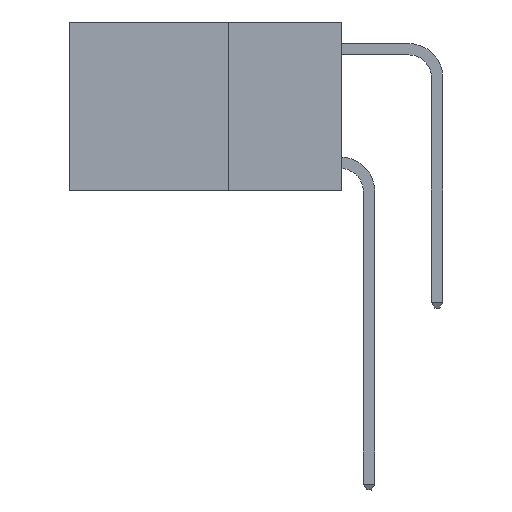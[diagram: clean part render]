
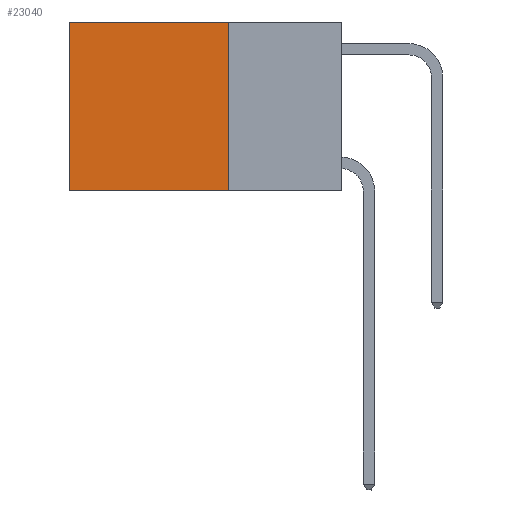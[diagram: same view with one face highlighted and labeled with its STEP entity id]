
A CAD part, left-side view. The second image highlights one B-rep face of the part: STEP entity #23040.
In plain terms, the highlighted planar face has unit normal (-1, 0, 0).
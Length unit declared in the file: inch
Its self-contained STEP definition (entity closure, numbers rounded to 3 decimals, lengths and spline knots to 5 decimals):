
#12 = VECTOR ( 'NONE', #2665, 39.37008 ) ;
#282 = ORIENTED_EDGE ( 'NONE', *, *, #5734, .F. ) ;
#461 = CARTESIAN_POINT ( 'NONE',  ( 0.2625, 0.25, 0. ) ) ;
#656 = CARTESIAN_POINT ( 'NONE',  ( 0.2625, 0.6, 0. ) ) ;
#1303 = LINE ( 'NONE', #15928, #11339 ) ;
#1490 = PLANE ( 'NONE',  #4434 ) ;
#1645 = DIRECTION ( 'NONE',  ( 0., 1., 0. ) ) ;
#2469 = DIRECTION ( 'NONE',  ( 0., 0., -1. ) ) ;
#2665 = DIRECTION ( 'NONE',  ( 0., 0., -1. ) ) ;
#3499 = DIRECTION ( 'NONE',  ( 1., 0., 0. ) ) ;
#4025 = LINE ( 'NONE', #25321, #8783 ) ;
#4434 = AXIS2_PLACEMENT_3D ( 'NONE', #15422, #3499, #17405 ) ;
#4719 = EDGE_CURVE ( 'NONE', #8634, #23724, #15917, .T. ) ;
#5163 = VECTOR ( 'NONE', #2469, 39.37008 ) ;
#5345 = CARTESIAN_POINT ( 'NONE',  ( 0.2625, 0.6, -0.37 ) ) ;
#5734 = EDGE_CURVE ( 'NONE', #16293, #23724, #4025, .T. ) ;
#6446 = LINE ( 'NONE', #461, #5163 ) ;
#8358 = EDGE_LOOP ( 'NONE', ( #12036, #282, #9505, #20150 ) ) ;
#8634 = VERTEX_POINT ( 'NONE', #14025 ) ;
#8783 = VECTOR ( 'NONE', #1645, 39.37008 ) ;
#9505 = ORIENTED_EDGE ( 'NONE', *, *, #22695, .F. ) ;
#11339 = VECTOR ( 'NONE', #13862, 39.37008 ) ;
#12036 = ORIENTED_EDGE ( 'NONE', *, *, #4719, .T. ) ;
#13862 = DIRECTION ( 'NONE',  ( 0., 1., 0. ) ) ;
#14025 = CARTESIAN_POINT ( 'NONE',  ( 0.2625, 0.6, 0. ) ) ;
#15032 = VERTEX_POINT ( 'NONE', #22337 ) ;
#15263 = CARTESIAN_POINT ( 'NONE',  ( 0.2625, 0.25, -0.37 ) ) ;
#15422 = CARTESIAN_POINT ( 'NONE',  ( 0.2625, 0.25, 0. ) ) ;
#15917 = LINE ( 'NONE', #656, #12 ) ;
#15928 = CARTESIAN_POINT ( 'NONE',  ( 0.2625, 0.25, 0. ) ) ;
#16293 = VERTEX_POINT ( 'NONE', #15263 ) ;
#17210 = EDGE_CURVE ( 'NONE', #15032, #8634, #1303, .T. ) ;
#17405 = DIRECTION ( 'NONE',  ( 0., 0., -1. ) ) ;
#20150 = ORIENTED_EDGE ( 'NONE', *, *, #17210, .T. ) ;
#22337 = CARTESIAN_POINT ( 'NONE',  ( 0.2625, 0.25, 0. ) ) ;
#22695 = EDGE_CURVE ( 'NONE', #15032, #16293, #6446, .T. ) ;
#23040 = ADVANCED_FACE ( 'NONE', ( #23966 ), #1490, .F. ) ;
#23724 = VERTEX_POINT ( 'NONE', #5345 ) ;
#23966 = FACE_OUTER_BOUND ( 'NONE', #8358, .T. ) ;
#25321 = CARTESIAN_POINT ( 'NONE',  ( 0.2625, 0.25, -0.37 ) ) ;
